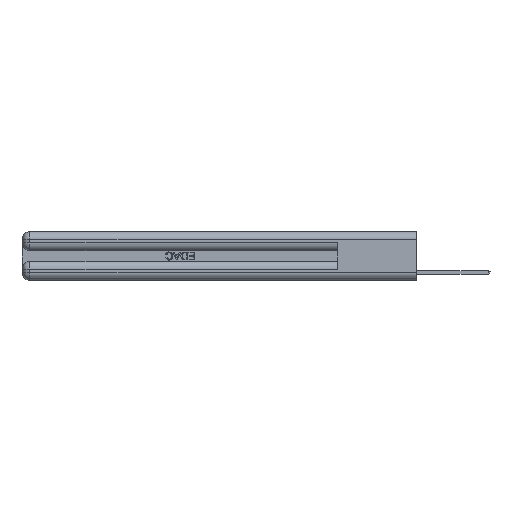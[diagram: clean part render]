
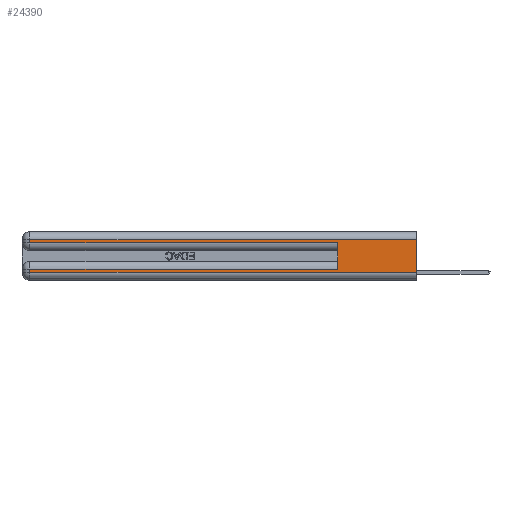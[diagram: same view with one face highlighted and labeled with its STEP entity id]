
A CAD part, left-side view. The second image highlights one B-rep face of the part: STEP entity #24390.
In plain terms, the highlighted planar face has unit normal (-1, 0, 0).
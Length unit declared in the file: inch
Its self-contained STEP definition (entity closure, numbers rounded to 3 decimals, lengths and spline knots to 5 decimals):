
#1951 = EDGE_CURVE ( 'NONE', #23017, #4807, #6488, .T. ) ;
#2297 = LINE ( 'NONE', #19987, #10441 ) ;
#2565 = CARTESIAN_POINT ( 'NONE',  ( 0., 0.6, 0.285 ) ) ;
#3353 = EDGE_CURVE ( 'NONE', #31078, #23017, #15305, .T. ) ;
#3361 = VECTOR ( 'NONE', #20103, 39.37008 ) ;
#3419 = ORIENTED_EDGE ( 'NONE', *, *, #1951, .T. ) ;
#4155 = DIRECTION ( 'NONE',  ( 0., 0., 1. ) ) ;
#4231 = CARTESIAN_POINT ( 'NONE',  ( 0., 0., 0.06 ) ) ;
#4807 = VERTEX_POINT ( 'NONE', #30432 ) ;
#4911 = DIRECTION ( 'NONE',  ( 0., 0., -1. ) ) ;
#5612 = VERTEX_POINT ( 'NONE', #2565 ) ;
#6488 = LINE ( 'NONE', #23386, #10416 ) ;
#6673 = ORIENTED_EDGE ( 'NONE', *, *, #10946, .F. ) ;
#6782 = VECTOR ( 'NONE', #4911, 39.37008 ) ;
#7340 = CARTESIAN_POINT ( 'NONE',  ( 0., 0.6, 0.085 ) ) ;
#7393 = VERTEX_POINT ( 'NONE', #27196 ) ;
#7743 = LINE ( 'NONE', #18415, #9665 ) ;
#9119 = VERTEX_POINT ( 'NONE', #18882 ) ;
#9389 = EDGE_CURVE ( 'NONE', #9119, #27406, #28166, .T. ) ;
#9568 = PLANE ( 'NONE',  #26907 ) ;
#9665 = VECTOR ( 'NONE', #4155, 39.37008 ) ;
#10416 = VECTOR ( 'NONE', #20709, 39.37008 ) ;
#10441 = VECTOR ( 'NONE', #12906, 39.37008 ) ;
#10784 = CARTESIAN_POINT ( 'NONE',  ( 0., 2.94, 0.285 ) ) ;
#10946 = EDGE_CURVE ( 'NONE', #31078, #5612, #7743, .T. ) ;
#11759 = VECTOR ( 'NONE', #17671, 39.37008 ) ;
#12062 = ORIENTED_EDGE ( 'NONE', *, *, #24125, .T. ) ;
#12636 = ORIENTED_EDGE ( 'NONE', *, *, #18813, .T. ) ;
#12906 = DIRECTION ( 'NONE',  ( 0., -1., 0. ) ) ;
#14084 = LINE ( 'NONE', #19593, #6782 ) ;
#14853 = VECTOR ( 'NONE', #28482, 39.37008 ) ;
#15305 = LINE ( 'NONE', #19684, #3361 ) ;
#15583 = CARTESIAN_POINT ( 'NONE',  ( 0., 2.94, 0.37 ) ) ;
#16434 = CARTESIAN_POINT ( 'NONE',  ( 0., 0., 0.37 ) ) ;
#17671 = DIRECTION ( 'NONE',  ( 0., 1., 0. ) ) ;
#18001 = ORIENTED_EDGE ( 'NONE', *, *, #9389, .T. ) ;
#18415 = CARTESIAN_POINT ( 'NONE',  ( 0., 0.6, 0.145 ) ) ;
#18813 = EDGE_CURVE ( 'NONE', #4807, #21710, #29764, .T. ) ;
#18882 = CARTESIAN_POINT ( 'NONE',  ( 0., 2.94, 0.31 ) ) ;
#19307 = DIRECTION ( 'NONE',  ( 1., 0., 0. ) ) ;
#19593 = CARTESIAN_POINT ( 'NONE',  ( 0., 0., 0.37 ) ) ;
#19684 = CARTESIAN_POINT ( 'NONE',  ( 0., 0., 0.085 ) ) ;
#19987 = CARTESIAN_POINT ( 'NONE',  ( 0., 0., 0.285 ) ) ;
#20103 = DIRECTION ( 'NONE',  ( 0., 1., 0. ) ) ;
#20466 = DIRECTION ( 'NONE',  ( 0., 0., -1. ) ) ;
#20709 = DIRECTION ( 'NONE',  ( 0., 0., -1. ) ) ;
#20853 = VECTOR ( 'NONE', #20466, 39.37008 ) ;
#21187 = EDGE_LOOP ( 'NONE', ( #29012, #31212, #18001, #12062, #6673, #24056, #3419, #12636 ) ) ;
#21414 = EDGE_CURVE ( 'NONE', #7393, #9119, #31289, .T. ) ;
#21710 = VERTEX_POINT ( 'NONE', #4231 ) ;
#22275 = FACE_OUTER_BOUND ( 'NONE', #21187, .T. ) ;
#22662 = CARTESIAN_POINT ( 'NONE',  ( 0., 0., 0.31 ) ) ;
#23017 = VERTEX_POINT ( 'NONE', #23425 ) ;
#23386 = CARTESIAN_POINT ( 'NONE',  ( 0., 2.94, 0.37 ) ) ;
#23425 = CARTESIAN_POINT ( 'NONE',  ( 0., 2.94, 0.085 ) ) ;
#24056 = ORIENTED_EDGE ( 'NONE', *, *, #3353, .T. ) ;
#24125 = EDGE_CURVE ( 'NONE', #27406, #5612, #2297, .T. ) ;
#24390 = ADVANCED_FACE ( 'NONE', ( #22275 ), #9568, .F. ) ;
#26425 = EDGE_CURVE ( 'NONE', #7393, #21710, #14084, .T. ) ;
#26683 = DIRECTION ( 'NONE',  ( 0., 0., -1. ) ) ;
#26907 = AXIS2_PLACEMENT_3D ( 'NONE', #16434, #19307, #26683 ) ;
#27196 = CARTESIAN_POINT ( 'NONE',  ( 0., 0., 0.31 ) ) ;
#27406 = VERTEX_POINT ( 'NONE', #10784 ) ;
#28063 = CARTESIAN_POINT ( 'NONE',  ( 0., 0., 0.06 ) ) ;
#28166 = LINE ( 'NONE', #15583, #20853 ) ;
#28482 = DIRECTION ( 'NONE',  ( 0., -1., 0. ) ) ;
#29012 = ORIENTED_EDGE ( 'NONE', *, *, #26425, .F. ) ;
#29764 = LINE ( 'NONE', #28063, #14853 ) ;
#30432 = CARTESIAN_POINT ( 'NONE',  ( 0., 2.94, 0.06 ) ) ;
#31078 = VERTEX_POINT ( 'NONE', #7340 ) ;
#31212 = ORIENTED_EDGE ( 'NONE', *, *, #21414, .T. ) ;
#31289 = LINE ( 'NONE', #22662, #11759 ) ;
